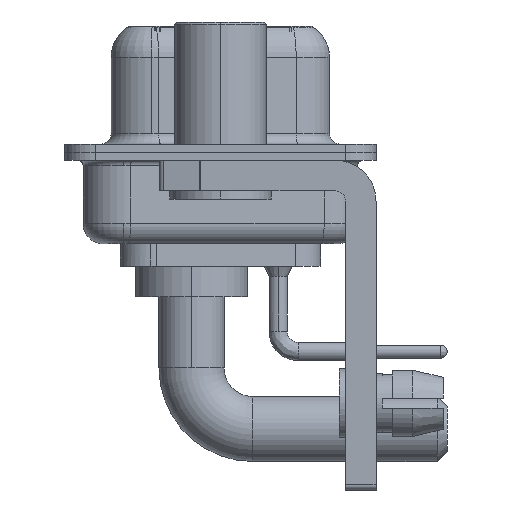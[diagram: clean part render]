
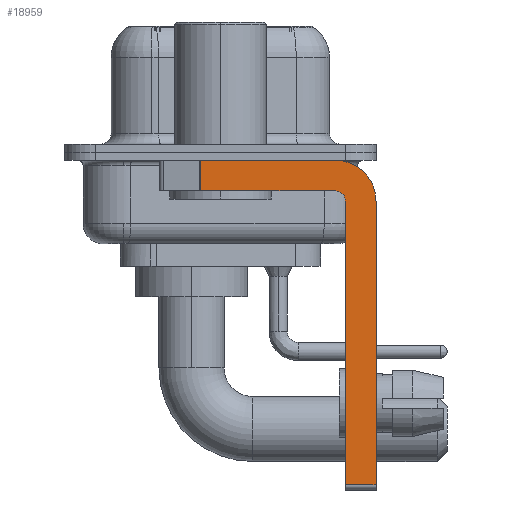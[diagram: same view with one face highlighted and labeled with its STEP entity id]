
A CAD part, left-side view. The second image highlights one B-rep face of the part: STEP entity #18959.
In plain terms, the highlighted planar face has unit normal (-1, 0, 0).
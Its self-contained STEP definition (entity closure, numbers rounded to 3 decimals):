
#269 = LINE ( 'NONE', #3667, #7109 ) ;
#327 = DIRECTION ( 'NONE',  ( 0., 0., -1. ) ) ;
#377 = PLANE ( 'NONE',  #4917 ) ;
#665 = AXIS2_PLACEMENT_3D ( 'NONE', #6157, #8510, #871 ) ;
#685 = CARTESIAN_POINT ( 'NONE',  ( -2.9, -5.65, -2.4 ) ) ;
#871 = DIRECTION ( 'NONE',  ( 0., 0., -1. ) ) ;
#1047 = DIRECTION ( 'NONE',  ( -1., 0., 0. ) ) ;
#2325 = CARTESIAN_POINT ( 'NONE',  ( -2.9, 0.978, -1.9 ) ) ;
#2441 = ORIENTED_EDGE ( 'NONE', *, *, #22038, .T. ) ;
#2485 = VECTOR ( 'NONE', #7620, 1000. ) ;
#2620 = FACE_OUTER_BOUND ( 'NONE', #22899, .T. ) ;
#3478 = CIRCLE ( 'NONE', #665, 2. ) ;
#3667 = CARTESIAN_POINT ( 'NONE',  ( -2.9, 3., -0.4 ) ) ;
#3753 = VECTOR ( 'NONE', #12166, 1000. ) ;
#3915 = VERTEX_POINT ( 'NONE', #23769 ) ;
#4058 = ORIENTED_EDGE ( 'NONE', *, *, #21233, .T. ) ;
#4917 = AXIS2_PLACEMENT_3D ( 'NONE', #6265, #18005, #23534 ) ;
#5139 = CARTESIAN_POINT ( 'NONE',  ( -2.9, 0.978, -1.9 ) ) ;
#6157 = CARTESIAN_POINT ( 'NONE',  ( -2.9, -5.65, -2.4 ) ) ;
#6240 = EDGE_CURVE ( 'NONE', #20970, #17026, #10692, .T. ) ;
#6265 = CARTESIAN_POINT ( 'NONE',  ( -2.9, -5.65, -2.4 ) ) ;
#7042 = DIRECTION ( 'NONE',  ( 0., -1., 0. ) ) ;
#7109 = VECTOR ( 'NONE', #9282, 1000. ) ;
#7441 = CARTESIAN_POINT ( 'NONE',  ( -2.9, 0.978, -0.4 ) ) ;
#7584 = VERTEX_POINT ( 'NONE', #8845 ) ;
#7620 = DIRECTION ( 'NONE',  ( 0., 0., 1. ) ) ;
#7717 = LINE ( 'NONE', #2325, #13020 ) ;
#8440 = DIRECTION ( 'NONE',  ( 0., 0., 1. ) ) ;
#8510 = DIRECTION ( 'NONE',  ( 1., 0., 0. ) ) ;
#8779 = CARTESIAN_POINT ( 'NONE',  ( -2.9, -5.65, -16.35 ) ) ;
#8845 = CARTESIAN_POINT ( 'NONE',  ( -2.9, -6.15, -16.35 ) ) ;
#9282 = DIRECTION ( 'NONE',  ( 0., -1., 0. ) ) ;
#9468 = EDGE_CURVE ( 'NONE', #23448, #23911, #16028, .T. ) ;
#9762 = CARTESIAN_POINT ( 'NONE',  ( -2.9, -5.65, -0.4 ) ) ;
#9964 = ORIENTED_EDGE ( 'NONE', *, *, #18288, .F. ) ;
#10367 = EDGE_CURVE ( 'NONE', #3915, #23448, #12563, .T. ) ;
#10692 = LINE ( 'NONE', #17742, #19266 ) ;
#12166 = DIRECTION ( 'NONE',  ( 0., 1., 0. ) ) ;
#12252 = ORIENTED_EDGE ( 'NONE', *, *, #23478, .F. ) ;
#12563 = CIRCLE ( 'NONE', #19750, 0.5 ) ;
#13020 = VECTOR ( 'NONE', #327, 1000. ) ;
#13067 = ORIENTED_EDGE ( 'NONE', *, *, #6240, .F. ) ;
#13429 = CARTESIAN_POINT ( 'NONE',  ( -2.9, -5.65, -1.9 ) ) ;
#14566 = ORIENTED_EDGE ( 'NONE', *, *, #10367, .F. ) ;
#15036 = VECTOR ( 'NONE', #7042, 1000. ) ;
#15299 = VERTEX_POINT ( 'NONE', #9762 ) ;
#15736 = DIRECTION ( 'NONE',  ( 0., 0., -1. ) ) ;
#16028 = LINE ( 'NONE', #23804, #3753 ) ;
#17026 = VERTEX_POINT ( 'NONE', #20986 ) ;
#17279 = ORIENTED_EDGE ( 'NONE', *, *, #9468, .F. ) ;
#17742 = CARTESIAN_POINT ( 'NONE',  ( -2.9, -7.65, -2.4 ) ) ;
#18005 = DIRECTION ( 'NONE',  ( 1., 0., 0. ) ) ;
#18288 = EDGE_CURVE ( 'NONE', #7584, #3915, #24263, .T. ) ;
#18959 = ADVANCED_FACE ( 'NONE', ( #2620 ), #377, .F. ) ;
#19266 = VECTOR ( 'NONE', #15736, 1000. ) ;
#19750 = AXIS2_PLACEMENT_3D ( 'NONE', #685, #1047, #8440 ) ;
#20230 = VERTEX_POINT ( 'NONE', #7441 ) ;
#20412 = LINE ( 'NONE', #8779, #15036 ) ;
#20731 = CARTESIAN_POINT ( 'NONE',  ( -2.9, -7.65, -2.4 ) ) ;
#20970 = VERTEX_POINT ( 'NONE', #20731 ) ;
#20986 = CARTESIAN_POINT ( 'NONE',  ( -2.9, -7.65, -16.35 ) ) ;
#21233 = EDGE_CURVE ( 'NONE', #20230, #23911, #7717, .T. ) ;
#22038 = EDGE_CURVE ( 'NONE', #7584, #17026, #20412, .T. ) ;
#22362 = ORIENTED_EDGE ( 'NONE', *, *, #23637, .F. ) ;
#22899 = EDGE_LOOP ( 'NONE', ( #12252, #4058, #17279, #14566, #9964, #2441, #13067, #22362 ) ) ;
#23448 = VERTEX_POINT ( 'NONE', #13429 ) ;
#23478 = EDGE_CURVE ( 'NONE', #20230, #15299, #269, .T. ) ;
#23534 = DIRECTION ( 'NONE',  ( 0., 0., -1. ) ) ;
#23637 = EDGE_CURVE ( 'NONE', #15299, #20970, #3478, .T. ) ;
#23769 = CARTESIAN_POINT ( 'NONE',  ( -2.9, -6.15, -2.4 ) ) ;
#23804 = CARTESIAN_POINT ( 'NONE',  ( -2.9, -5.65, -1.9 ) ) ;
#23911 = VERTEX_POINT ( 'NONE', #5139 ) ;
#24263 = LINE ( 'NONE', #24388, #2485 ) ;
#24388 = CARTESIAN_POINT ( 'NONE',  ( -2.9, -6.15, -16.6 ) ) ;
